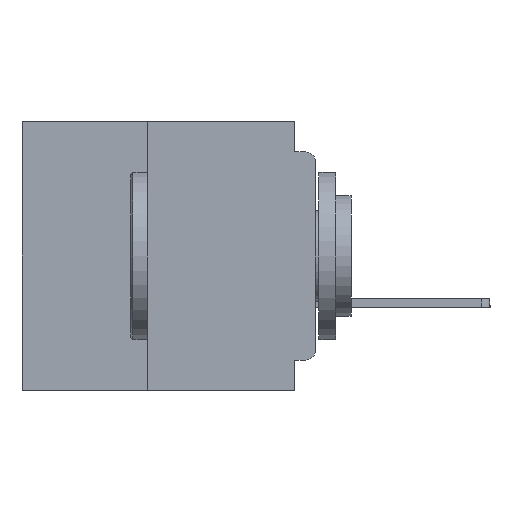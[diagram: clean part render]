
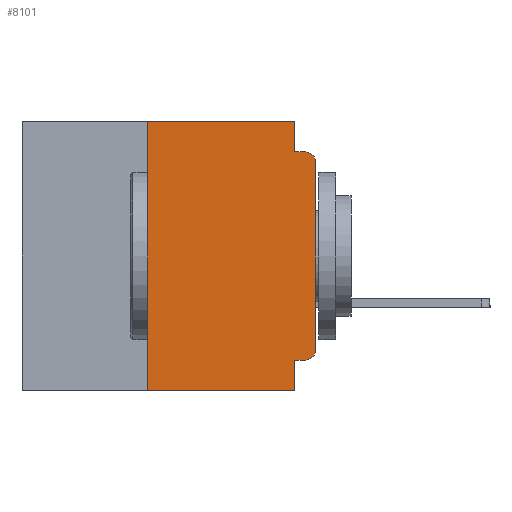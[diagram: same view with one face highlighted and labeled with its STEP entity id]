
A CAD part, left-side view. The second image highlights one B-rep face of the part: STEP entity #8101.
In plain terms, the highlighted planar face has unit normal (-1, 0, 0).
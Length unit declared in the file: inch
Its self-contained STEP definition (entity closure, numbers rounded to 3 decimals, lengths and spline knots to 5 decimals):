
#141 = CARTESIAN_POINT ( 'NONE',  ( 0., 0.031, -0.4 ) ) ;
#2045 = DIRECTION ( 'NONE',  ( 1., 0., 0. ) ) ;
#2365 = EDGE_CURVE ( 'NONE', #4247, #49065, #26916, .T. ) ;
#2749 = EDGE_LOOP ( 'NONE', ( #53140, #7586, #51514, #39044, #55522, #43614, #14241, #55684, #45278, #36823 ) ) ;
#4105 = DIRECTION ( 'NONE',  ( 0., 0., -1. ) ) ;
#4247 = VERTEX_POINT ( 'NONE', #56619 ) ;
#4390 = DIRECTION ( 'NONE',  ( 0., 0., 1. ) ) ;
#5972 = EDGE_CURVE ( 'NONE', #26297, #4247, #57065, .T. ) ;
#6910 = VECTOR ( 'NONE', #52277, 39.37008 ) ;
#7298 = DIRECTION ( 'NONE',  ( -1., 0., 0. ) ) ;
#7385 = DIRECTION ( 'NONE',  ( 0., 1., 0. ) ) ;
#7586 = ORIENTED_EDGE ( 'NONE', *, *, #41942, .T. ) ;
#8101 = ADVANCED_FACE ( 'NONE', ( #59334 ), #12646, .F. ) ;
#9759 = CARTESIAN_POINT ( 'NONE',  ( 0., 0.031, -0.355 ) ) ;
#10160 = EDGE_CURVE ( 'NONE', #22580, #25230, #24561, .T. ) ;
#10294 = AXIS2_PLACEMENT_3D ( 'NONE', #55408, #2045, #39623 ) ;
#10987 = VECTOR ( 'NONE', #40056, 39.37008 ) ;
#12646 = PLANE ( 'NONE',  #10294 ) ;
#13431 = CARTESIAN_POINT ( 'NONE',  ( 0., 0., -0.045 ) ) ;
#13435 = DIRECTION ( 'NONE',  ( 0., 0., 1. ) ) ;
#13872 = CARTESIAN_POINT ( 'NONE',  ( 0., 0., -0.34 ) ) ;
#13954 = CARTESIAN_POINT ( 'NONE',  ( 0., 0.031, 0. ) ) ;
#14241 = ORIENTED_EDGE ( 'NONE', *, *, #41320, .T. ) ;
#14739 = DIRECTION ( 'NONE',  ( -1., 0., 0. ) ) ;
#14848 = CARTESIAN_POINT ( 'NONE',  ( 0., 0.031, -0.045 ) ) ;
#15824 = VERTEX_POINT ( 'NONE', #36970 ) ;
#17969 = DIRECTION ( 'NONE',  ( 0., -1., 0. ) ) ;
#19178 = EDGE_CURVE ( 'NONE', #21474, #35580, #20793, .T. ) ;
#19299 = AXIS2_PLACEMENT_3D ( 'NONE', #39451, #7298, #44810 ) ;
#20793 = LINE ( 'NONE', #13431, #47603 ) ;
#21474 = VERTEX_POINT ( 'NONE', #14848 ) ;
#22580 = VERTEX_POINT ( 'NONE', #9759 ) ;
#24561 = LINE ( 'NONE', #68293, #6910 ) ;
#25230 = VERTEX_POINT ( 'NONE', #141 ) ;
#25698 = EDGE_CURVE ( 'NONE', #15824, #40014, #38652, .T. ) ;
#26297 = VERTEX_POINT ( 'NONE', #30559 ) ;
#26916 = LINE ( 'NONE', #46123, #10987 ) ;
#30559 = CARTESIAN_POINT ( 'NONE',  ( 0., 0.25, -0.4 ) ) ;
#31854 = LINE ( 'NONE', #33924, #44411 ) ;
#33096 = LINE ( 'NONE', #44660, #43948 ) ;
#33924 = CARTESIAN_POINT ( 'NONE',  ( 0., 0.437, -0.4 ) ) ;
#35019 = CARTESIAN_POINT ( 'NONE',  ( 0., 0.25, -0.4 ) ) ;
#35580 = VERTEX_POINT ( 'NONE', #37548 ) ;
#36823 = ORIENTED_EDGE ( 'NONE', *, *, #25698, .T. ) ;
#36970 = CARTESIAN_POINT ( 'NONE',  ( 0., 0.015, -0.355 ) ) ;
#37548 = CARTESIAN_POINT ( 'NONE',  ( 0., 0.015, -0.045 ) ) ;
#38652 = CIRCLE ( 'NONE', #54092, 0.015 ) ;
#38682 = VERTEX_POINT ( 'NONE', #55348 ) ;
#39044 = ORIENTED_EDGE ( 'NONE', *, *, #52436, .F. ) ;
#39451 = CARTESIAN_POINT ( 'NONE',  ( 0., 0.015, -0.06 ) ) ;
#39623 = DIRECTION ( 'NONE',  ( 0., 0., -1. ) ) ;
#39918 = VECTOR ( 'NONE', #4105, 39.37008 ) ;
#40014 = VERTEX_POINT ( 'NONE', #13872 ) ;
#40056 = DIRECTION ( 'NONE',  ( 0., -1., 0. ) ) ;
#40153 = DIRECTION ( 'NONE',  ( 0., -1., 0. ) ) ;
#41320 = EDGE_CURVE ( 'NONE', #26297, #25230, #31854, .T. ) ;
#41641 = CARTESIAN_POINT ( 'NONE',  ( 0., 0.031, 0. ) ) ;
#41942 = EDGE_CURVE ( 'NONE', #38682, #35580, #46833, .T. ) ;
#43614 = ORIENTED_EDGE ( 'NONE', *, *, #5972, .F. ) ;
#43948 = VECTOR ( 'NONE', #7385, 39.37008 ) ;
#44411 = VECTOR ( 'NONE', #17969, 39.37008 ) ;
#44660 = CARTESIAN_POINT ( 'NONE',  ( 0., 0., -0.355 ) ) ;
#44810 = DIRECTION ( 'NONE',  ( 0., 0., -1. ) ) ;
#44950 = EDGE_CURVE ( 'NONE', #15824, #22580, #33096, .T. ) ;
#45278 = ORIENTED_EDGE ( 'NONE', *, *, #44950, .F. ) ;
#46123 = CARTESIAN_POINT ( 'NONE',  ( 0., 0.437, 0. ) ) ;
#46451 = EDGE_CURVE ( 'NONE', #40014, #38682, #60194, .T. ) ;
#46782 = CARTESIAN_POINT ( 'NONE',  ( 0., 0.015, -0.34 ) ) ;
#46833 = CIRCLE ( 'NONE', #19299, 0.015 ) ;
#47603 = VECTOR ( 'NONE', #40153, 39.37008 ) ;
#49065 = VERTEX_POINT ( 'NONE', #13954 ) ;
#51514 = ORIENTED_EDGE ( 'NONE', *, *, #19178, .F. ) ;
#52111 = DIRECTION ( 'NONE',  ( 0., 0., -1. ) ) ;
#52277 = DIRECTION ( 'NONE',  ( 0., 0., -1. ) ) ;
#52436 = EDGE_CURVE ( 'NONE', #49065, #21474, #68181, .T. ) ;
#53140 = ORIENTED_EDGE ( 'NONE', *, *, #46451, .T. ) ;
#54092 = AXIS2_PLACEMENT_3D ( 'NONE', #46782, #14739, #52111 ) ;
#55348 = CARTESIAN_POINT ( 'NONE',  ( 0., 0., -0.06 ) ) ;
#55408 = CARTESIAN_POINT ( 'NONE',  ( 0., 0.437, 0. ) ) ;
#55522 = ORIENTED_EDGE ( 'NONE', *, *, #2365, .F. ) ;
#55684 = ORIENTED_EDGE ( 'NONE', *, *, #10160, .F. ) ;
#56619 = CARTESIAN_POINT ( 'NONE',  ( 0., 0.25, 0. ) ) ;
#57065 = LINE ( 'NONE', #35019, #58722 ) ;
#58722 = VECTOR ( 'NONE', #13435, 39.37008 ) ;
#59334 = FACE_OUTER_BOUND ( 'NONE', #2749, .T. ) ;
#60194 = LINE ( 'NONE', #68175, #69347 ) ;
#68175 = CARTESIAN_POINT ( 'NONE',  ( 0., 0., 0. ) ) ;
#68181 = LINE ( 'NONE', #41641, #39918 ) ;
#68293 = CARTESIAN_POINT ( 'NONE',  ( 0., 0.031, -0.4 ) ) ;
#69347 = VECTOR ( 'NONE', #4390, 39.37008 ) ;
